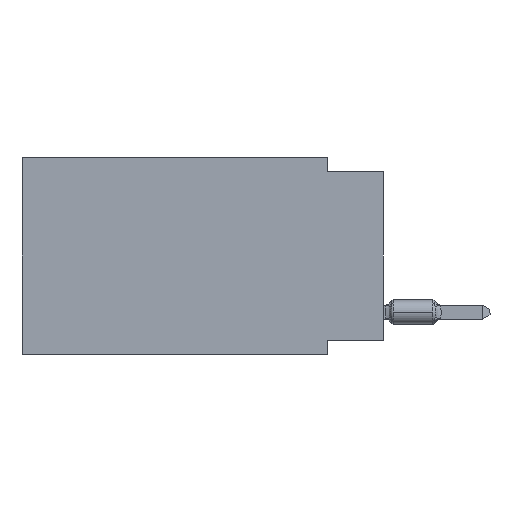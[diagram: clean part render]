
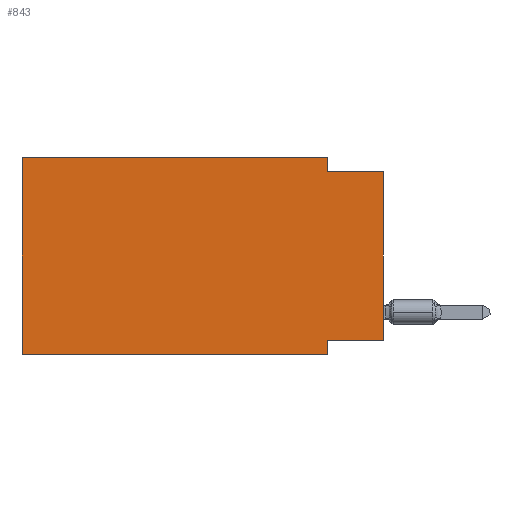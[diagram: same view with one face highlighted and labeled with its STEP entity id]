
A CAD part, left-side view. The second image highlights one B-rep face of the part: STEP entity #843.
In plain terms, the highlighted planar face has unit normal (-1, 0, 0).
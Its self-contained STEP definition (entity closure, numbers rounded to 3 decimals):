
#89 = PLANE ( 'NONE',  #5437 ) ;
#437 = VERTEX_POINT ( 'NONE', #2232 ) ;
#439 = VECTOR ( 'NONE', #7777, 1000. ) ;
#775 = VERTEX_POINT ( 'NONE', #6554 ) ;
#843 = ADVANCED_FACE ( 'NONE', ( #10573 ), #89, .F. ) ;
#914 = EDGE_CURVE ( 'NONE', #3239, #775, #2808, .T. ) ;
#1357 = CARTESIAN_POINT ( 'NONE',  ( 0., 16.383, -8.89 ) ) ;
#1612 = ORIENTED_EDGE ( 'NONE', *, *, #10533, .F. ) ;
#1627 = ORIENTED_EDGE ( 'NONE', *, *, #914, .T. ) ;
#1802 = LINE ( 'NONE', #3710, #11231 ) ;
#2092 = EDGE_CURVE ( 'NONE', #6563, #775, #7028, .T. ) ;
#2193 = CARTESIAN_POINT ( 'NONE',  ( 0., 2.54, -0.635 ) ) ;
#2202 = DIRECTION ( 'NONE',  ( 0., 0., -1. ) ) ;
#2232 = CARTESIAN_POINT ( 'NONE',  ( 0., 16.383, 0. ) ) ;
#2633 = CARTESIAN_POINT ( 'NONE',  ( 0., 0., -8.255 ) ) ;
#2808 = LINE ( 'NONE', #7981, #439 ) ;
#3049 = VECTOR ( 'NONE', #10255, 1000. ) ;
#3097 = ORIENTED_EDGE ( 'NONE', *, *, #8933, .F. ) ;
#3171 = DIRECTION ( 'NONE',  ( 0., 0., 1. ) ) ;
#3216 = VECTOR ( 'NONE', #9958, 1000. ) ;
#3239 = VERTEX_POINT ( 'NONE', #2633 ) ;
#3252 = EDGE_CURVE ( 'NONE', #8677, #6563, #11351, .T. ) ;
#3291 = DIRECTION ( 'NONE',  ( 1., 0., 0. ) ) ;
#3630 = DIRECTION ( 'NONE',  ( 0., -1., 0. ) ) ;
#3710 = CARTESIAN_POINT ( 'NONE',  ( 0., 2.54, -8.89 ) ) ;
#3922 = LINE ( 'NONE', #3991, #5723 ) ;
#3972 = CARTESIAN_POINT ( 'NONE',  ( 0., 0., -0.635 ) ) ;
#3991 = CARTESIAN_POINT ( 'NONE',  ( 0., 16.383, 0. ) ) ;
#4260 = EDGE_LOOP ( 'NONE', ( #1627, #9668, #12493, #8349, #7442, #5208, #3097, #1612 ) ) ;
#4790 = EDGE_CURVE ( 'NONE', #11191, #437, #3922, .T. ) ;
#5208 = ORIENTED_EDGE ( 'NONE', *, *, #6888, .T. ) ;
#5437 = AXIS2_PLACEMENT_3D ( 'NONE', #12549, #3291, #2202 ) ;
#5723 = VECTOR ( 'NONE', #3171, 1000. ) ;
#6065 = CARTESIAN_POINT ( 'NONE',  ( 0., 16.383, -8.89 ) ) ;
#6554 = CARTESIAN_POINT ( 'NONE',  ( 0., 0., -0.635 ) ) ;
#6563 = VERTEX_POINT ( 'NONE', #2193 ) ;
#6888 = EDGE_CURVE ( 'NONE', #11191, #7180, #12394, .T. ) ;
#7028 = LINE ( 'NONE', #3972, #12645 ) ;
#7180 = VERTEX_POINT ( 'NONE', #9998 ) ;
#7442 = ORIENTED_EDGE ( 'NONE', *, *, #4790, .F. ) ;
#7777 = DIRECTION ( 'NONE',  ( 0., 0., 1. ) ) ;
#7981 = CARTESIAN_POINT ( 'NONE',  ( 0., 0., 0. ) ) ;
#8349 = ORIENTED_EDGE ( 'NONE', *, *, #10556, .F. ) ;
#8391 = VECTOR ( 'NONE', #10283, 1000. ) ;
#8677 = VERTEX_POINT ( 'NONE', #13386 ) ;
#8741 = LINE ( 'NONE', #10090, #11910 ) ;
#8866 = CARTESIAN_POINT ( 'NONE',  ( 0., 0., -8.255 ) ) ;
#8933 = EDGE_CURVE ( 'NONE', #11622, #7180, #1802, .T. ) ;
#8964 = CARTESIAN_POINT ( 'NONE',  ( 0., 2.54, 0. ) ) ;
#9025 = DIRECTION ( 'NONE',  ( 0., 0., -1. ) ) ;
#9668 = ORIENTED_EDGE ( 'NONE', *, *, #2092, .F. ) ;
#9958 = DIRECTION ( 'NONE',  ( 0., 1., 0. ) ) ;
#9998 = CARTESIAN_POINT ( 'NONE',  ( 0., 2.54, -8.89 ) ) ;
#10090 = CARTESIAN_POINT ( 'NONE',  ( 0., 16.383, 0. ) ) ;
#10255 = DIRECTION ( 'NONE',  ( 0., 0., -1. ) ) ;
#10283 = DIRECTION ( 'NONE',  ( 0., -1., 0. ) ) ;
#10533 = EDGE_CURVE ( 'NONE', #3239, #11622, #12127, .T. ) ;
#10556 = EDGE_CURVE ( 'NONE', #437, #8677, #8741, .T. ) ;
#10573 = FACE_OUTER_BOUND ( 'NONE', #4260, .T. ) ;
#11191 = VERTEX_POINT ( 'NONE', #1357 ) ;
#11231 = VECTOR ( 'NONE', #9025, 1000. ) ;
#11351 = LINE ( 'NONE', #8964, #3049 ) ;
#11389 = DIRECTION ( 'NONE',  ( 0., -1., 0. ) ) ;
#11487 = CARTESIAN_POINT ( 'NONE',  ( 0., 2.54, -8.255 ) ) ;
#11622 = VERTEX_POINT ( 'NONE', #11487 ) ;
#11910 = VECTOR ( 'NONE', #3630, 1000. ) ;
#12127 = LINE ( 'NONE', #8866, #3216 ) ;
#12394 = LINE ( 'NONE', #6065, #8391 ) ;
#12493 = ORIENTED_EDGE ( 'NONE', *, *, #3252, .F. ) ;
#12549 = CARTESIAN_POINT ( 'NONE',  ( 0., 16.383, 0. ) ) ;
#12645 = VECTOR ( 'NONE', #11389, 1000. ) ;
#13386 = CARTESIAN_POINT ( 'NONE',  ( 0., 2.54, 0. ) ) ;
